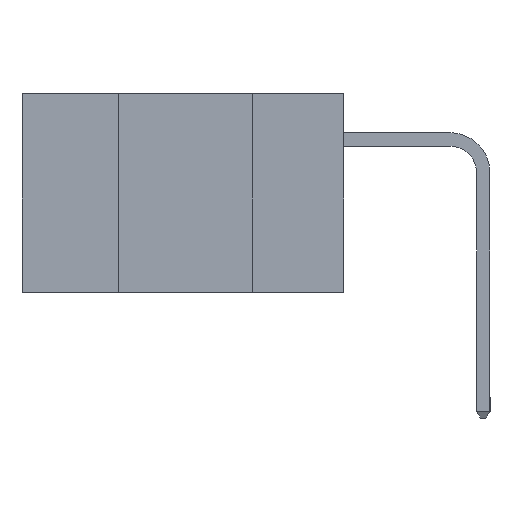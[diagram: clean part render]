
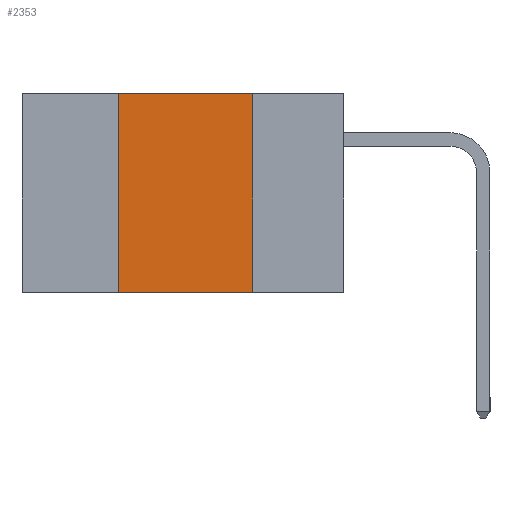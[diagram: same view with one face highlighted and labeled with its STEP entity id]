
A CAD part, left-side view. The second image highlights one B-rep face of the part: STEP entity #2353.
In plain terms, the highlighted planar face has unit normal (-1, 0, 0).
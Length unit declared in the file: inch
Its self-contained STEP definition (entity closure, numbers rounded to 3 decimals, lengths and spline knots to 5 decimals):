
#840 = DIRECTION ( 'NONE',  ( 0., 0., -1. ) ) ;
#1452 = LINE ( 'NONE', #19419, #12991 ) ;
#2353 = ADVANCED_FACE ( 'NONE', ( #18380 ), #7333, .F. ) ;
#2556 = LINE ( 'NONE', #9399, #15034 ) ;
#3343 = CARTESIAN_POINT ( 'NONE',  ( 0., 0.17, -0.37 ) ) ;
#3904 = DIRECTION ( 'NONE',  ( 0., 0., -1. ) ) ;
#5879 = DIRECTION ( 'NONE',  ( 0., -1., 0. ) ) ;
#6109 = EDGE_CURVE ( 'NONE', #19010, #20011, #16802, .T. ) ;
#6262 = VECTOR ( 'NONE', #5879, 39.37008 ) ;
#6545 = ORIENTED_EDGE ( 'NONE', *, *, #6109, .F. ) ;
#7333 = PLANE ( 'NONE',  #12822 ) ;
#7788 = EDGE_LOOP ( 'NONE', ( #14292, #6545, #11592, #16408 ) ) ;
#8629 = VECTOR ( 'NONE', #19619, 39.37008 ) ;
#9399 = CARTESIAN_POINT ( 'NONE',  ( 0., 0.42, -0.37 ) ) ;
#9930 = LINE ( 'NONE', #15160, #6262 ) ;
#10386 = VERTEX_POINT ( 'NONE', #3343 ) ;
#10680 = VERTEX_POINT ( 'NONE', #11973 ) ;
#10894 = EDGE_CURVE ( 'NONE', #10680, #19010, #2556, .T. ) ;
#11592 = ORIENTED_EDGE ( 'NONE', *, *, #10894, .F. ) ;
#11748 = EDGE_CURVE ( 'NONE', #10680, #10386, #9930, .T. ) ;
#11973 = CARTESIAN_POINT ( 'NONE',  ( 0., 0.42, -0.37 ) ) ;
#12822 = AXIS2_PLACEMENT_3D ( 'NONE', #17465, #13304, #3904 ) ;
#12991 = VECTOR ( 'NONE', #840, 39.37008 ) ;
#13304 = DIRECTION ( 'NONE',  ( 1., 0., 0. ) ) ;
#13514 = EDGE_CURVE ( 'NONE', #20011, #10386, #1452, .T. ) ;
#13837 = CARTESIAN_POINT ( 'NONE',  ( 0., 0.17, 0. ) ) ;
#14292 = ORIENTED_EDGE ( 'NONE', *, *, #13514, .F. ) ;
#15034 = VECTOR ( 'NONE', #18577, 39.37008 ) ;
#15160 = CARTESIAN_POINT ( 'NONE',  ( 0., 0.6, -0.37 ) ) ;
#16408 = ORIENTED_EDGE ( 'NONE', *, *, #11748, .T. ) ;
#16802 = LINE ( 'NONE', #20087, #8629 ) ;
#17465 = CARTESIAN_POINT ( 'NONE',  ( 0., 0.6, 0. ) ) ;
#18380 = FACE_OUTER_BOUND ( 'NONE', #7788, .T. ) ;
#18577 = DIRECTION ( 'NONE',  ( 0., 0., 1. ) ) ;
#19010 = VERTEX_POINT ( 'NONE', #19315 ) ;
#19315 = CARTESIAN_POINT ( 'NONE',  ( 0., 0.42, 0. ) ) ;
#19419 = CARTESIAN_POINT ( 'NONE',  ( 0., 0.17, -0.37 ) ) ;
#19619 = DIRECTION ( 'NONE',  ( 0., -1., 0. ) ) ;
#20011 = VERTEX_POINT ( 'NONE', #13837 ) ;
#20087 = CARTESIAN_POINT ( 'NONE',  ( 0., 0.6, 0. ) ) ;
